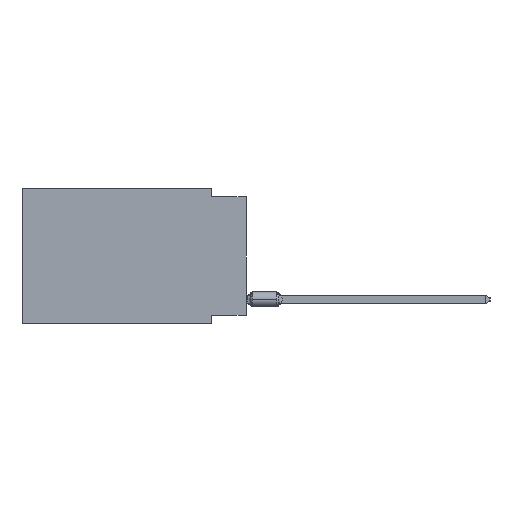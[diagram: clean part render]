
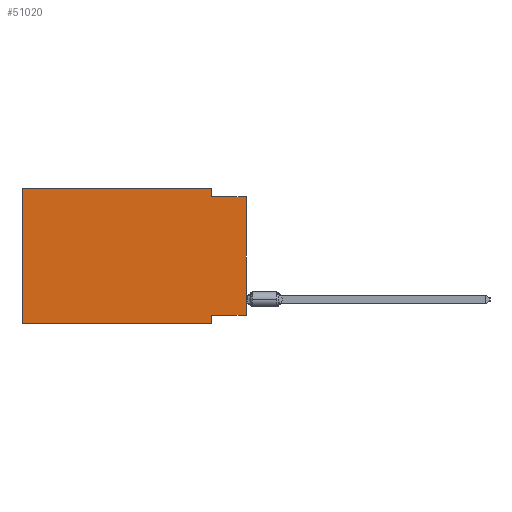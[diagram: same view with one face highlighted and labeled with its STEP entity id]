
A CAD part, left-side view. The second image highlights one B-rep face of the part: STEP entity #51020.
In plain terms, the highlighted planar face has unit normal (-1, 0, 0).
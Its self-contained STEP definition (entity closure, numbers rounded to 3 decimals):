
#1415 = ORIENTED_EDGE ( 'NONE', *, *, #10940, .F. ) ;
#2097 = FACE_OUTER_BOUND ( 'NONE', #3886, .T. ) ;
#2385 = EDGE_CURVE ( 'NONE', #17794, #14287, #35936, .T. ) ;
#2390 = DIRECTION ( 'NONE',  ( 1., 0., 0. ) ) ;
#2616 = LINE ( 'NONE', #16335, #5254 ) ;
#2769 = DIRECTION ( 'NONE',  ( 0., 0., 1. ) ) ;
#3886 = EDGE_LOOP ( 'NONE', ( #54362, #26702, #1415, #43006, #53652, #20195, #27213, #8326 ) ) ;
#5254 = VECTOR ( 'NONE', #37816, 1000. ) ;
#7353 = CARTESIAN_POINT ( 'NONE',  ( 0., 16.383, 0. ) ) ;
#7399 = CARTESIAN_POINT ( 'NONE',  ( 0., 2.54, -9.271 ) ) ;
#8326 = ORIENTED_EDGE ( 'NONE', *, *, #37603, .F. ) ;
#8707 = VECTOR ( 'NONE', #49444, 1000. ) ;
#10197 = CARTESIAN_POINT ( 'NONE',  ( 0., 0., -0.635 ) ) ;
#10479 = DIRECTION ( 'NONE',  ( 0., -1., 0. ) ) ;
#10517 = VERTEX_POINT ( 'NONE', #21881 ) ;
#10940 = EDGE_CURVE ( 'NONE', #10517, #17794, #49264, .T. ) ;
#13743 = EDGE_CURVE ( 'NONE', #22719, #31887, #52849, .T. ) ;
#14287 = VERTEX_POINT ( 'NONE', #15701 ) ;
#15701 = CARTESIAN_POINT ( 'NONE',  ( 0., 0., -0.635 ) ) ;
#16335 = CARTESIAN_POINT ( 'NONE',  ( 0., 0., 0. ) ) ;
#16978 = LINE ( 'NONE', #48169, #42714 ) ;
#17091 = CARTESIAN_POINT ( 'NONE',  ( 0., 2.54, -0.635 ) ) ;
#17462 = VECTOR ( 'NONE', #36945, 1000. ) ;
#17527 = DIRECTION ( 'NONE',  ( 0., 1., 0. ) ) ;
#17794 = VERTEX_POINT ( 'NONE', #17091 ) ;
#18403 = VECTOR ( 'NONE', #37580, 1000. ) ;
#18916 = CARTESIAN_POINT ( 'NONE',  ( 0., 2.54, 0. ) ) ;
#19021 = VERTEX_POINT ( 'NONE', #7399 ) ;
#19835 = DIRECTION ( 'NONE',  ( 0., 0., -1. ) ) ;
#20195 = ORIENTED_EDGE ( 'NONE', *, *, #13743, .T. ) ;
#21283 = VERTEX_POINT ( 'NONE', #38917 ) ;
#21823 = AXIS2_PLACEMENT_3D ( 'NONE', #41593, #2390, #19835 ) ;
#21881 = CARTESIAN_POINT ( 'NONE',  ( 0., 2.54, 0. ) ) ;
#22516 = CARTESIAN_POINT ( 'NONE',  ( 0., 16.383, -9.906 ) ) ;
#22719 = VERTEX_POINT ( 'NONE', #51597 ) ;
#26702 = ORIENTED_EDGE ( 'NONE', *, *, #2385, .F. ) ;
#27213 = ORIENTED_EDGE ( 'NONE', *, *, #35764, .F. ) ;
#27874 = VECTOR ( 'NONE', #53418, 1000. ) ;
#28525 = LINE ( 'NONE', #7353, #48789 ) ;
#30643 = CARTESIAN_POINT ( 'NONE',  ( 0., 0., -9.271 ) ) ;
#31887 = VERTEX_POINT ( 'NONE', #51060 ) ;
#32326 = VECTOR ( 'NONE', #10479, 1000. ) ;
#32533 = LINE ( 'NONE', #50010, #8707 ) ;
#33669 = EDGE_CURVE ( 'NONE', #22719, #21283, #28525, .T. ) ;
#35764 = EDGE_CURVE ( 'NONE', #19021, #31887, #32533, .T. ) ;
#35936 = LINE ( 'NONE', #10197, #32326 ) ;
#36945 = DIRECTION ( 'NONE',  ( 0., 0., -1. ) ) ;
#37580 = DIRECTION ( 'NONE',  ( 0., -1., 0. ) ) ;
#37603 = EDGE_CURVE ( 'NONE', #46203, #19021, #16978, .T. ) ;
#37816 = DIRECTION ( 'NONE',  ( 0., 0., 1. ) ) ;
#37865 = CARTESIAN_POINT ( 'NONE',  ( 0., 16.383, 0. ) ) ;
#38917 = CARTESIAN_POINT ( 'NONE',  ( 0., 16.383, 0. ) ) ;
#41593 = CARTESIAN_POINT ( 'NONE',  ( 0., 16.383, 0. ) ) ;
#42336 = EDGE_CURVE ( 'NONE', #21283, #10517, #42725, .T. ) ;
#42714 = VECTOR ( 'NONE', #17527, 1000. ) ;
#42725 = LINE ( 'NONE', #37865, #18403 ) ;
#43006 = ORIENTED_EDGE ( 'NONE', *, *, #42336, .F. ) ;
#45901 = PLANE ( 'NONE',  #21823 ) ;
#46203 = VERTEX_POINT ( 'NONE', #30643 ) ;
#48169 = CARTESIAN_POINT ( 'NONE',  ( 0., 0., -9.271 ) ) ;
#48789 = VECTOR ( 'NONE', #2769, 1000. ) ;
#49264 = LINE ( 'NONE', #18916, #17462 ) ;
#49444 = DIRECTION ( 'NONE',  ( 0., 0., -1. ) ) ;
#50010 = CARTESIAN_POINT ( 'NONE',  ( 0., 2.54, -9.906 ) ) ;
#51020 = ADVANCED_FACE ( 'NONE', ( #2097 ), #45901, .F. ) ;
#51060 = CARTESIAN_POINT ( 'NONE',  ( 0., 2.54, -9.906 ) ) ;
#51597 = CARTESIAN_POINT ( 'NONE',  ( 0., 16.383, -9.906 ) ) ;
#52849 = LINE ( 'NONE', #22516, #27874 ) ;
#53418 = DIRECTION ( 'NONE',  ( 0., -1., 0. ) ) ;
#53652 = ORIENTED_EDGE ( 'NONE', *, *, #33669, .F. ) ;
#54362 = ORIENTED_EDGE ( 'NONE', *, *, #56465, .T. ) ;
#56465 = EDGE_CURVE ( 'NONE', #46203, #14287, #2616, .T. ) ;
